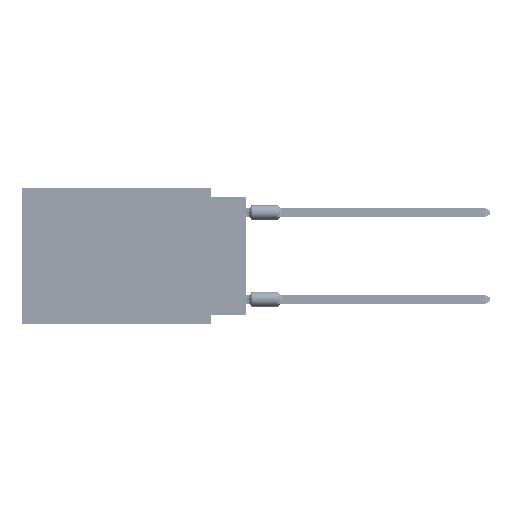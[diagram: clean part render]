
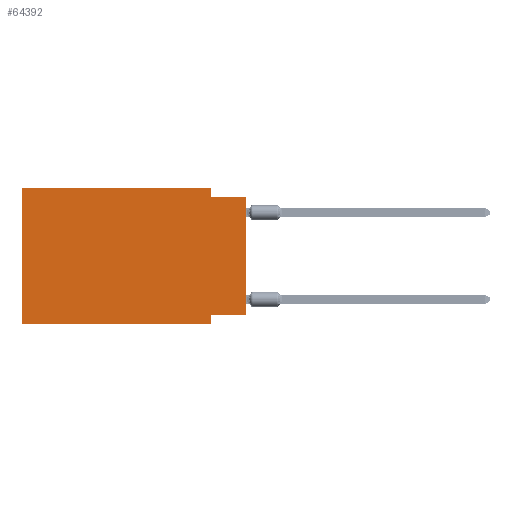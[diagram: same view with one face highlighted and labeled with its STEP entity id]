
A CAD part, left-side view. The second image highlights one B-rep face of the part: STEP entity #64392.
In plain terms, the highlighted planar face has unit normal (-1, 0, 0).
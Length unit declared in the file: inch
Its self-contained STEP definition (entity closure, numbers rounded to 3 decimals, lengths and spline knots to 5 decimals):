
#2108 = EDGE_CURVE ( 'NONE', #68120, #15485, #65228, .T. ) ;
#3177 = DIRECTION ( 'NONE',  ( 0., 0., -1. ) ) ;
#4442 = VECTOR ( 'NONE', #29591, 39.37008 ) ;
#7859 = VERTEX_POINT ( 'NONE', #60603 ) ;
#8890 = DIRECTION ( 'NONE',  ( 0., 0., -1. ) ) ;
#9003 = CARTESIAN_POINT ( 'NONE',  ( 0., 0., -0.365 ) ) ;
#10174 = DIRECTION ( 'NONE',  ( 1., 0., 0. ) ) ;
#11343 = CARTESIAN_POINT ( 'NONE',  ( 0., 0., -0.025 ) ) ;
#12539 = ORIENTED_EDGE ( 'NONE', *, *, #2108, .T. ) ;
#13472 = EDGE_CURVE ( 'NONE', #30491, #15485, #48634, .T. ) ;
#15485 = VERTEX_POINT ( 'NONE', #20827 ) ;
#16384 = LINE ( 'NONE', #30001, #4442 ) ;
#17957 = VECTOR ( 'NONE', #21051, 39.37008 ) ;
#19042 = EDGE_LOOP ( 'NONE', ( #34192, #59079, #63034, #46538, #77968, #12539, #46719, #49438 ) ) ;
#20827 = CARTESIAN_POINT ( 'NONE',  ( 0., 0.1, -0.39 ) ) ;
#20985 = DIRECTION ( 'NONE',  ( 0., 1., 0. ) ) ;
#21051 = DIRECTION ( 'NONE',  ( 0., -1., 0. ) ) ;
#21772 = FACE_OUTER_BOUND ( 'NONE', #19042, .T. ) ;
#23340 = EDGE_CURVE ( 'NONE', #68120, #59165, #16384, .T. ) ;
#23942 = VERTEX_POINT ( 'NONE', #32707 ) ;
#28145 = EDGE_CURVE ( 'NONE', #45599, #47756, #48102, .T. ) ;
#28760 = EDGE_CURVE ( 'NONE', #45599, #30491, #64346, .T. ) ;
#29591 = DIRECTION ( 'NONE',  ( 0., 0., 1. ) ) ;
#30001 = CARTESIAN_POINT ( 'NONE',  ( 0., 0.645, 0. ) ) ;
#30491 = VERTEX_POINT ( 'NONE', #60913 ) ;
#30692 = LINE ( 'NONE', #44606, #32733 ) ;
#32707 = CARTESIAN_POINT ( 'NONE',  ( 0., 0.1, 0. ) ) ;
#32733 = VECTOR ( 'NONE', #62057, 39.37008 ) ;
#34192 = ORIENTED_EDGE ( 'NONE', *, *, #28145, .T. ) ;
#38038 = CARTESIAN_POINT ( 'NONE',  ( 0., 0.645, -0.39 ) ) ;
#38312 = CARTESIAN_POINT ( 'NONE',  ( 0., 0., -0.365 ) ) ;
#39970 = CARTESIAN_POINT ( 'NONE',  ( 0., 0.645, 0. ) ) ;
#40269 = VECTOR ( 'NONE', #49047, 39.37008 ) ;
#42414 = VECTOR ( 'NONE', #8890, 39.37008 ) ;
#44606 = CARTESIAN_POINT ( 'NONE',  ( 0., 0.645, 0. ) ) ;
#45599 = VERTEX_POINT ( 'NONE', #38312 ) ;
#45764 = VECTOR ( 'NONE', #20985, 39.37008 ) ;
#46538 = ORIENTED_EDGE ( 'NONE', *, *, #50755, .F. ) ;
#46719 = ORIENTED_EDGE ( 'NONE', *, *, #13472, .F. ) ;
#46901 = CARTESIAN_POINT ( 'NONE',  ( 0., 0.1, 0. ) ) ;
#47601 = CARTESIAN_POINT ( 'NONE',  ( 0., 0., -0.025 ) ) ;
#47756 = VERTEX_POINT ( 'NONE', #47601 ) ;
#48102 = LINE ( 'NONE', #73304, #78835 ) ;
#48634 = LINE ( 'NONE', #60613, #40269 ) ;
#49047 = DIRECTION ( 'NONE',  ( 0., 0., -1. ) ) ;
#49438 = ORIENTED_EDGE ( 'NONE', *, *, #28760, .F. ) ;
#50755 = EDGE_CURVE ( 'NONE', #59165, #23942, #30692, .T. ) ;
#53559 = PLANE ( 'NONE',  #53794 ) ;
#53794 = AXIS2_PLACEMENT_3D ( 'NONE', #39970, #10174, #3177 ) ;
#54651 = EDGE_CURVE ( 'NONE', #7859, #47756, #67937, .T. ) ;
#58263 = CARTESIAN_POINT ( 'NONE',  ( 0., 0.645, 0. ) ) ;
#58642 = CARTESIAN_POINT ( 'NONE',  ( 0., 0.645, -0.39 ) ) ;
#59079 = ORIENTED_EDGE ( 'NONE', *, *, #54651, .F. ) ;
#59165 = VERTEX_POINT ( 'NONE', #58263 ) ;
#60603 = CARTESIAN_POINT ( 'NONE',  ( 0., 0.1, -0.025 ) ) ;
#60613 = CARTESIAN_POINT ( 'NONE',  ( 0., 0.1, -0.39 ) ) ;
#60913 = CARTESIAN_POINT ( 'NONE',  ( 0., 0.1, -0.365 ) ) ;
#61720 = DIRECTION ( 'NONE',  ( 0., -1., 0. ) ) ;
#62057 = DIRECTION ( 'NONE',  ( 0., -1., 0. ) ) ;
#63034 = ORIENTED_EDGE ( 'NONE', *, *, #70306, .F. ) ;
#64346 = LINE ( 'NONE', #9003, #45764 ) ;
#64392 = ADVANCED_FACE ( 'NONE', ( #21772 ), #53559, .F. ) ;
#65228 = LINE ( 'NONE', #58642, #17957 ) ;
#65458 = LINE ( 'NONE', #46901, #42414 ) ;
#67937 = LINE ( 'NONE', #11343, #76467 ) ;
#68120 = VERTEX_POINT ( 'NONE', #38038 ) ;
#70306 = EDGE_CURVE ( 'NONE', #23942, #7859, #65458, .T. ) ;
#73304 = CARTESIAN_POINT ( 'NONE',  ( 0., 0., 0. ) ) ;
#76467 = VECTOR ( 'NONE', #61720, 39.37008 ) ;
#77968 = ORIENTED_EDGE ( 'NONE', *, *, #23340, .F. ) ;
#78835 = VECTOR ( 'NONE', #79494, 39.37008 ) ;
#79494 = DIRECTION ( 'NONE',  ( 0., 0., 1. ) ) ;
